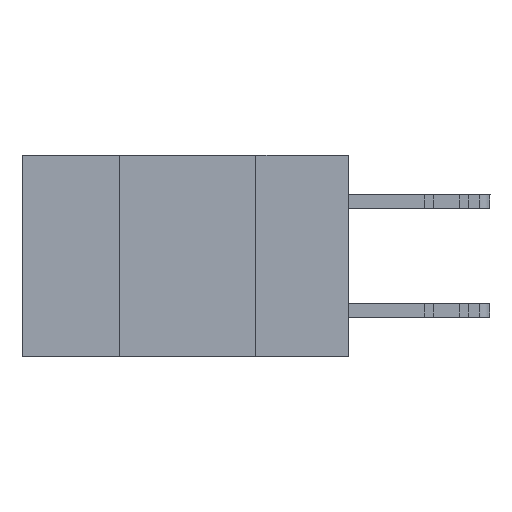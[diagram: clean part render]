
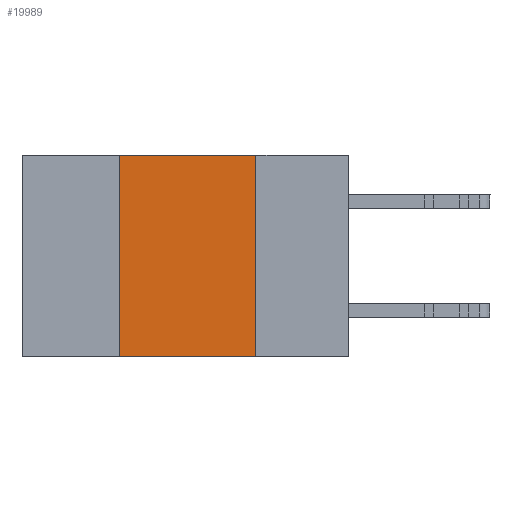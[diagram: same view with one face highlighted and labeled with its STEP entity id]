
A CAD part, left-side view. The second image highlights one B-rep face of the part: STEP entity #19989.
In plain terms, the highlighted planar face has unit normal (-1, 0, 0).
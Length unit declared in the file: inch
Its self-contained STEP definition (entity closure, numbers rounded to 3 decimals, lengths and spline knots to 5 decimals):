
#1996 = PLANE ( 'NONE',  #10112 ) ;
#2255 = VERTEX_POINT ( 'NONE', #23849 ) ;
#2384 = DIRECTION ( 'NONE',  ( 0., 0., 1. ) ) ;
#3408 = ORIENTED_EDGE ( 'NONE', *, *, #13099, .T. ) ;
#5766 = DIRECTION ( 'NONE',  ( 0., 0., -1. ) ) ;
#6878 = LINE ( 'NONE', #11392, #20658 ) ;
#7044 = EDGE_CURVE ( 'NONE', #17445, #20814, #8102, .T. ) ;
#8102 = LINE ( 'NONE', #27086, #26227 ) ;
#9448 = VECTOR ( 'NONE', #14880, 39.37008 ) ;
#10112 = AXIS2_PLACEMENT_3D ( 'NONE', #20961, #27826, #25196 ) ;
#10772 = CARTESIAN_POINT ( 'NONE',  ( 0., 0.17, -0.37 ) ) ;
#11392 = CARTESIAN_POINT ( 'NONE',  ( 0., 0.6, -0.37 ) ) ;
#13099 = EDGE_CURVE ( 'NONE', #2255, #20814, #6878, .T. ) ;
#13207 = FACE_OUTER_BOUND ( 'NONE', #17883, .T. ) ;
#13245 = CARTESIAN_POINT ( 'NONE',  ( 0., 0.42, 0. ) ) ;
#14880 = DIRECTION ( 'NONE',  ( 0., -1., 0. ) ) ;
#16904 = CARTESIAN_POINT ( 'NONE',  ( 0., 0.6, 0. ) ) ;
#17445 = VERTEX_POINT ( 'NONE', #29324 ) ;
#17883 = EDGE_LOOP ( 'NONE', ( #18803, #29088, #20842, #3408 ) ) ;
#18803 = ORIENTED_EDGE ( 'NONE', *, *, #7044, .F. ) ;
#19852 = LINE ( 'NONE', #16904, #9448 ) ;
#19989 = ADVANCED_FACE ( 'NONE', ( #13207 ), #1996, .F. ) ;
#20658 = VECTOR ( 'NONE', #26335, 39.37008 ) ;
#20814 = VERTEX_POINT ( 'NONE', #10772 ) ;
#20842 = ORIENTED_EDGE ( 'NONE', *, *, #30429, .F. ) ;
#20961 = CARTESIAN_POINT ( 'NONE',  ( 0., 0.6, 0. ) ) ;
#21929 = VECTOR ( 'NONE', #2384, 39.37008 ) ;
#23685 = LINE ( 'NONE', #25856, #21929 ) ;
#23849 = CARTESIAN_POINT ( 'NONE',  ( 0., 0.42, -0.37 ) ) ;
#25196 = DIRECTION ( 'NONE',  ( 0., 0., -1. ) ) ;
#25856 = CARTESIAN_POINT ( 'NONE',  ( 0., 0.42, 0. ) ) ;
#26227 = VECTOR ( 'NONE', #5766, 39.37008 ) ;
#26335 = DIRECTION ( 'NONE',  ( 0., -1., 0. ) ) ;
#26600 = VERTEX_POINT ( 'NONE', #13245 ) ;
#27086 = CARTESIAN_POINT ( 'NONE',  ( 0., 0.17, 0. ) ) ;
#27826 = DIRECTION ( 'NONE',  ( 1., 0., 0. ) ) ;
#28611 = EDGE_CURVE ( 'NONE', #26600, #17445, #19852, .T. ) ;
#29088 = ORIENTED_EDGE ( 'NONE', *, *, #28611, .F. ) ;
#29324 = CARTESIAN_POINT ( 'NONE',  ( 0., 0.17, 0. ) ) ;
#30429 = EDGE_CURVE ( 'NONE', #2255, #26600, #23685, .T. ) ;
